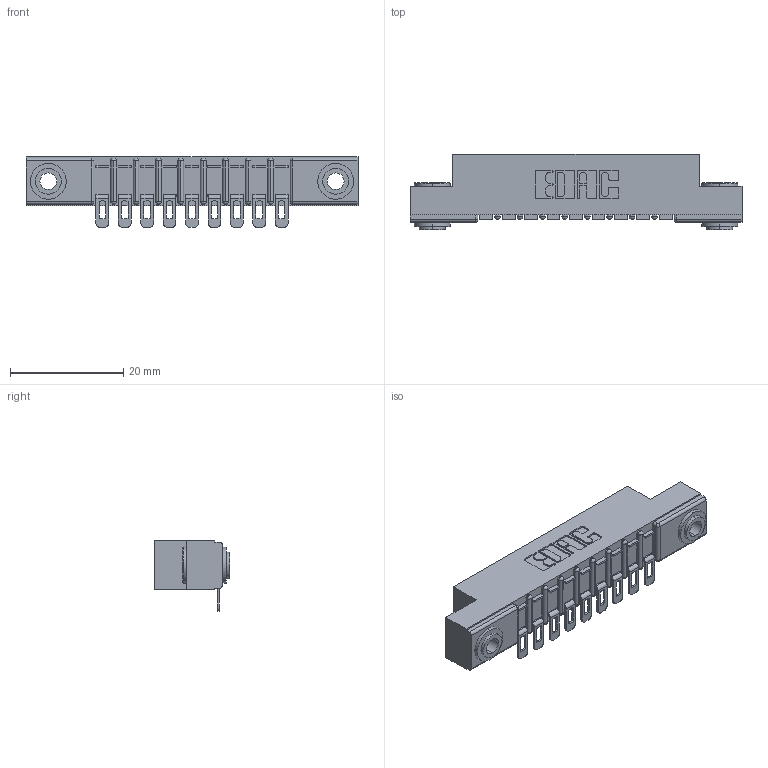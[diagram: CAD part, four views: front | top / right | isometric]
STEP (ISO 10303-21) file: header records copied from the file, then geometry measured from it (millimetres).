
FILE_DESCRIPTION (( 'STEP AP203' ), '1' );
FILE_NAME ('307-009-454-103.STEP', '2020-09-25T06:22:25', ( '' ), ( '' ), 'SwSTEP 2.0', 'SolidWorks 2020', '' );
FILE_SCHEMA (( 'CONFIG_CONTROL_DESIGN' ));
Length unit declared in the file: inch
Products named in the file (4): 307 Part_.156 Dia Mounting Holes; 345-250-002_345-250-002-102; 307-009-454-103; 307-290-002_554
Assembly tree (12 placements, depth 2):
  307-009-454-103
    307 Part_.156 Dia Mounting Holes
    307-290-002_554  x9
    345-250-002_345-250-002-102  x2
Bounding box: 58.67 x 13.36 x 12.52 mm (x, y, z)
Volume: 3871.3 mm3; surface area: 6599.3 mm2
Topology: 12 solids, 12 shells, 909 faces, 2712 edges, 1776 vertices
Faces by surface type: plane 508, cylinder 373, sphere 20, cone 8
Entity records: 13814 total; most frequent: CARTESIAN_POINT 2303, ORIENTED_EDGE 2284, DIRECTION 2274, EDGE_CURVE 1142, VECTOR 844, LINE 844, VERTEX_POINT 744, AXIS2_PLACEMENT_3D 715
